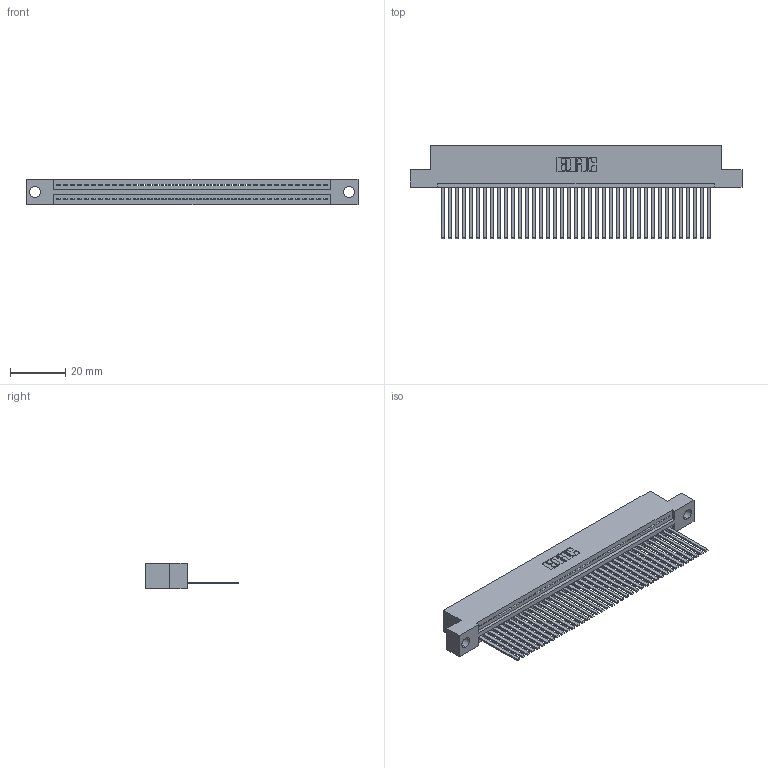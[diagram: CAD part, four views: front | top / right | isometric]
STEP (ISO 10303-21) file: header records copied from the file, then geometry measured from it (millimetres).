
FILE_DESCRIPTION (( 'STEP AP203' ), '1' );
FILE_NAME ('395-039-544-104.STEP', '2019-10-22T03:42:53', ( '' ), ( '' ), 'SwSTEP 2.0', 'SolidWorks 2016', '' );
FILE_SCHEMA (( 'CONFIG_CONTROL_DESIGN' ));
Length unit declared in the file: inch
Products named in the file (3): 395-039-544-104; 345-292-001_345-293-144; 345 Part_Flush Mounting Lugs - 0.156 Dia-TH
Assembly tree (40 placements, depth 2):
  395-039-544-104
    345 Part_Flush Mounting Lugs - 0.156 Dia-TH
    345-292-001_345-293-144  x39
Bounding box: 120.27 x 33.96 x 9.4 mm (x, y, z)
Volume: 11762.5 mm3; surface area: 16755.3 mm2
Topology: 40 solids, 40 shells, 2154 faces, 6503 edges, 4282 vertices
Faces by surface type: plane 1484, cylinder 670
Entity records: 29575 total; most frequent: CARTESIAN_POINT 5129, ORIENTED_EDGE 5102, DIRECTION 4481, EDGE_CURVE 2551, LINE 2267, VECTOR 2267, VERTEX_POINT 1698, AXIS2_PLACEMENT_3D 1107
